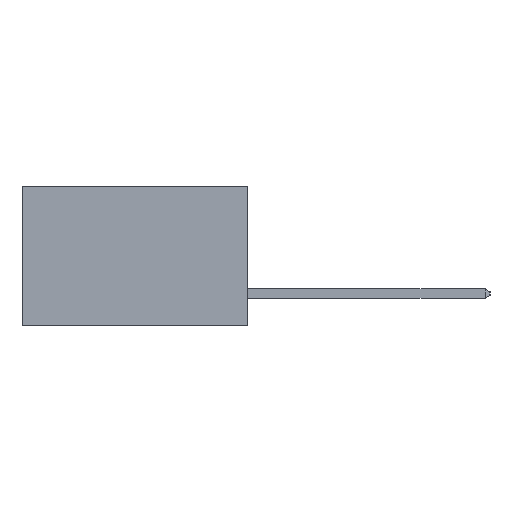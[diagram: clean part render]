
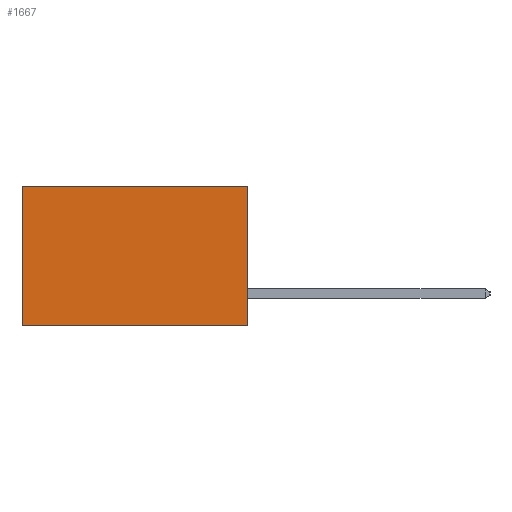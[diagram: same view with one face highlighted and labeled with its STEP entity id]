
A CAD part, left-side view. The second image highlights one B-rep face of the part: STEP entity #1667.
In plain terms, the highlighted planar face has unit normal (-1, 0, 0).
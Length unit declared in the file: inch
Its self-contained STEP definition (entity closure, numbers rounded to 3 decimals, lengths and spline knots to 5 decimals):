
#56 = CARTESIAN_POINT ( 'NONE',  ( 0.298, 0.6, -0.37 ) ) ;
#470 = DIRECTION ( 'NONE',  ( 0., 0., -1. ) ) ;
#522 = CARTESIAN_POINT ( 'NONE',  ( 0.298, 0.6, 0. ) ) ;
#918 = EDGE_CURVE ( 'NONE', #16081, #22542, #18797, .T. ) ;
#1667 = ADVANCED_FACE ( 'NONE', ( #5068 ), #14964, .F. ) ;
#1950 = EDGE_LOOP ( 'NONE', ( #5310, #9396, #15904, #24549 ) ) ;
#4307 = VECTOR ( 'NONE', #21952, 39.37008 ) ;
#4539 = EDGE_CURVE ( 'NONE', #26147, #5772, #4557, .T. ) ;
#4557 = LINE ( 'NONE', #25750, #9868 ) ;
#5068 = FACE_OUTER_BOUND ( 'NONE', #1950, .T. ) ;
#5310 = ORIENTED_EDGE ( 'NONE', *, *, #918, .T. ) ;
#5772 = VERTEX_POINT ( 'NONE', #9257 ) ;
#6388 = DIRECTION ( 'NONE',  ( 1., 0., 0. ) ) ;
#7566 = VECTOR ( 'NONE', #470, 39.37008 ) ;
#7734 = DIRECTION ( 'NONE',  ( 0., 1., 0. ) ) ;
#9257 = CARTESIAN_POINT ( 'NONE',  ( 0.298, 0., -0.37 ) ) ;
#9396 = ORIENTED_EDGE ( 'NONE', *, *, #24263, .F. ) ;
#9868 = VECTOR ( 'NONE', #25905, 39.37008 ) ;
#11040 = DIRECTION ( 'NONE',  ( 0., 0., -1. ) ) ;
#11971 = CARTESIAN_POINT ( 'NONE',  ( 0.298, 0., 0. ) ) ;
#14964 = PLANE ( 'NONE',  #17254 ) ;
#15904 = ORIENTED_EDGE ( 'NONE', *, *, #4539, .F. ) ;
#16081 = VERTEX_POINT ( 'NONE', #19327 ) ;
#16264 = LINE ( 'NONE', #19713, #4307 ) ;
#17254 = AXIS2_PLACEMENT_3D ( 'NONE', #28447, #6388, #11040 ) ;
#18797 = LINE ( 'NONE', #522, #7566 ) ;
#19224 = EDGE_CURVE ( 'NONE', #26147, #16081, #27117, .T. ) ;
#19327 = CARTESIAN_POINT ( 'NONE',  ( 0.298, 0.6, 0. ) ) ;
#19713 = CARTESIAN_POINT ( 'NONE',  ( 0.298, 0., -0.37 ) ) ;
#21952 = DIRECTION ( 'NONE',  ( 0., 1., 0. ) ) ;
#22150 = VECTOR ( 'NONE', #7734, 39.37008 ) ;
#22542 = VERTEX_POINT ( 'NONE', #56 ) ;
#23304 = CARTESIAN_POINT ( 'NONE',  ( 0.298, 0., 0. ) ) ;
#24263 = EDGE_CURVE ( 'NONE', #5772, #22542, #16264, .T. ) ;
#24549 = ORIENTED_EDGE ( 'NONE', *, *, #19224, .T. ) ;
#25750 = CARTESIAN_POINT ( 'NONE',  ( 0.298, 0., 0. ) ) ;
#25905 = DIRECTION ( 'NONE',  ( 0., 0., -1. ) ) ;
#26147 = VERTEX_POINT ( 'NONE', #11971 ) ;
#27117 = LINE ( 'NONE', #23304, #22150 ) ;
#28447 = CARTESIAN_POINT ( 'NONE',  ( 0.298, 0., 0. ) ) ;
